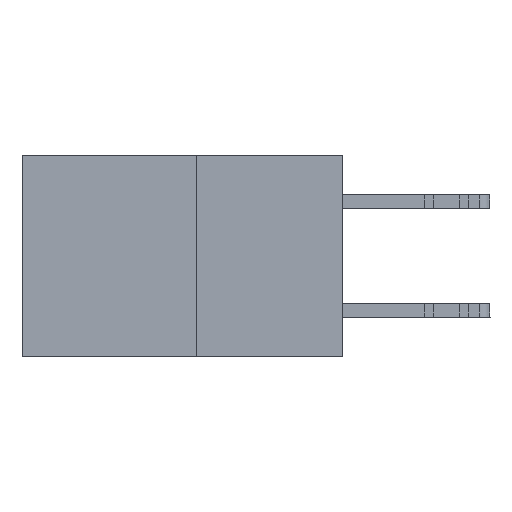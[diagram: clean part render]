
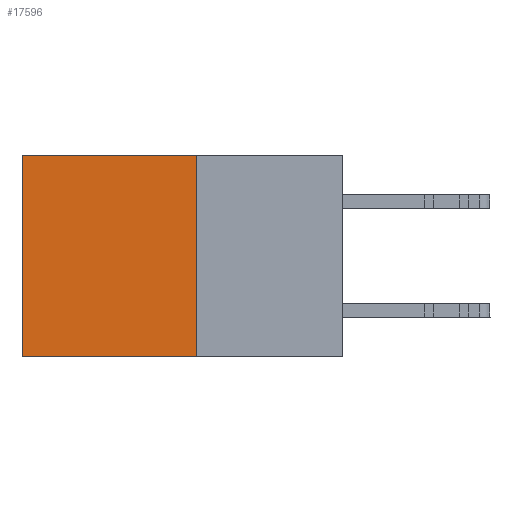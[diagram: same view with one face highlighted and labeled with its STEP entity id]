
A CAD part, left-side view. The second image highlights one B-rep face of the part: STEP entity #17596.
In plain terms, the highlighted planar face has unit normal (-1, 0, 0).
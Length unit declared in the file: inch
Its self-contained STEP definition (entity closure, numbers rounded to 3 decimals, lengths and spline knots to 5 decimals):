
#525 = CARTESIAN_POINT ( 'NONE',  ( 0.277, 0.27, 0. ) ) ;
#2087 = PLANE ( 'NONE',  #16488 ) ;
#2999 = FACE_OUTER_BOUND ( 'NONE', #17503, .T. ) ;
#3497 = VECTOR ( 'NONE', #24175, 39.37008 ) ;
#4744 = DIRECTION ( 'NONE',  ( 0., 0., -1. ) ) ;
#4859 = DIRECTION ( 'NONE',  ( 0., 0., -1. ) ) ;
#4987 = DIRECTION ( 'NONE',  ( 0., 0., -1. ) ) ;
#5008 = VERTEX_POINT ( 'NONE', #25823 ) ;
#5443 = ORIENTED_EDGE ( 'NONE', *, *, #7545, .F. ) ;
#5516 = VERTEX_POINT ( 'NONE', #15236 ) ;
#7343 = ORIENTED_EDGE ( 'NONE', *, *, #16449, .T. ) ;
#7545 = EDGE_CURVE ( 'NONE', #8251, #5008, #17287, .T. ) ;
#8251 = VERTEX_POINT ( 'NONE', #12550 ) ;
#9183 = VECTOR ( 'NONE', #4987, 39.37008 ) ;
#10005 = LINE ( 'NONE', #23215, #9183 ) ;
#10365 = VECTOR ( 'NONE', #24768, 39.37008 ) ;
#10907 = VECTOR ( 'NONE', #4859, 39.37008 ) ;
#12213 = LINE ( 'NONE', #525, #3497 ) ;
#12537 = LINE ( 'NONE', #28256, #10907 ) ;
#12550 = CARTESIAN_POINT ( 'NONE',  ( 0.277, 0.27, -0.37 ) ) ;
#13230 = EDGE_CURVE ( 'NONE', #5516, #5008, #10005, .T. ) ;
#15236 = CARTESIAN_POINT ( 'NONE',  ( 0.277, 0.59, 0. ) ) ;
#16449 = EDGE_CURVE ( 'NONE', #17015, #5516, #12213, .T. ) ;
#16488 = AXIS2_PLACEMENT_3D ( 'NONE', #17817, #20402, #4744 ) ;
#17015 = VERTEX_POINT ( 'NONE', #23555 ) ;
#17287 = LINE ( 'NONE', #24331, #10365 ) ;
#17503 = EDGE_LOOP ( 'NONE', ( #29807, #5443, #17916, #7343 ) ) ;
#17596 = ADVANCED_FACE ( 'NONE', ( #2999 ), #2087, .F. ) ;
#17817 = CARTESIAN_POINT ( 'NONE',  ( 0.277, 0.27, -0.37 ) ) ;
#17916 = ORIENTED_EDGE ( 'NONE', *, *, #20561, .F. ) ;
#20402 = DIRECTION ( 'NONE',  ( 1., 0., 0. ) ) ;
#20561 = EDGE_CURVE ( 'NONE', #17015, #8251, #12537, .T. ) ;
#23215 = CARTESIAN_POINT ( 'NONE',  ( 0.277, 0.59, -0.37 ) ) ;
#23555 = CARTESIAN_POINT ( 'NONE',  ( 0.277, 0.27, 0. ) ) ;
#24175 = DIRECTION ( 'NONE',  ( 0., 1., 0. ) ) ;
#24331 = CARTESIAN_POINT ( 'NONE',  ( 0.277, 0.27, -0.37 ) ) ;
#24768 = DIRECTION ( 'NONE',  ( 0., 1., 0. ) ) ;
#25823 = CARTESIAN_POINT ( 'NONE',  ( 0.277, 0.59, -0.37 ) ) ;
#28256 = CARTESIAN_POINT ( 'NONE',  ( 0.277, 0.27, -0.37 ) ) ;
#29807 = ORIENTED_EDGE ( 'NONE', *, *, #13230, .T. ) ;
